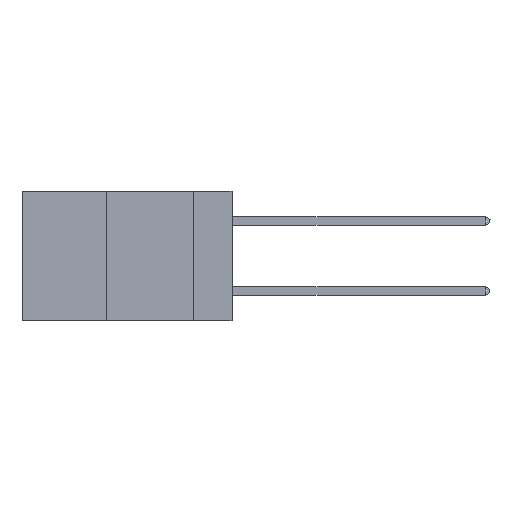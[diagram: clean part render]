
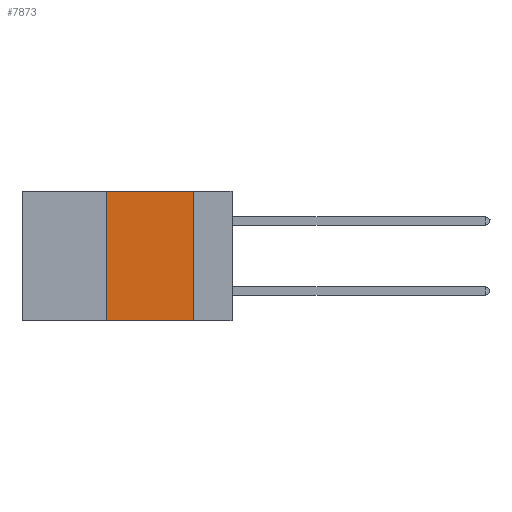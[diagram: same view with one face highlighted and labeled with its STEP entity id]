
A CAD part, left-side view. The second image highlights one B-rep face of the part: STEP entity #7873.
In plain terms, the highlighted planar face has unit normal (-1, 0, 0).
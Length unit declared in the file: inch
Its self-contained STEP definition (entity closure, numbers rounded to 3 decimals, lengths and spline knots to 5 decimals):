
#1733 = FACE_OUTER_BOUND ( 'NONE', #18670, .T. ) ;
#2161 = EDGE_CURVE ( 'NONE', #10029, #17665, #4350, .T. ) ;
#2415 = CARTESIAN_POINT ( 'NONE',  ( 0., 0.36, 0. ) ) ;
#2503 = VECTOR ( 'NONE', #9986, 39.37008 ) ;
#3212 = EDGE_CURVE ( 'NONE', #19777, #14713, #19995, .T. ) ;
#4350 = LINE ( 'NONE', #12884, #15622 ) ;
#5806 = LINE ( 'NONE', #18628, #14796 ) ;
#6129 = CARTESIAN_POINT ( 'NONE',  ( 0., 0.11, 0. ) ) ;
#6777 = CARTESIAN_POINT ( 'NONE',  ( 0., 0.11, 0. ) ) ;
#7456 = DIRECTION ( 'NONE',  ( 0., -1., 0. ) ) ;
#7873 = ADVANCED_FACE ( 'NONE', ( #1733 ), #9247, .F. ) ;
#9103 = ORIENTED_EDGE ( 'NONE', *, *, #13889, .T. ) ;
#9142 = CARTESIAN_POINT ( 'NONE',  ( 0., 0.6, -0.37 ) ) ;
#9247 = PLANE ( 'NONE',  #9894 ) ;
#9363 = EDGE_CURVE ( 'NONE', #17665, #19777, #5806, .T. ) ;
#9862 = ORIENTED_EDGE ( 'NONE', *, *, #3212, .F. ) ;
#9894 = AXIS2_PLACEMENT_3D ( 'NONE', #20603, #20751, #19154 ) ;
#9986 = DIRECTION ( 'NONE',  ( 0., 0., -1. ) ) ;
#9998 = LINE ( 'NONE', #9142, #17915 ) ;
#10029 = VERTEX_POINT ( 'NONE', #16297 ) ;
#12884 = CARTESIAN_POINT ( 'NONE',  ( 0., 0.36, 0. ) ) ;
#13889 = EDGE_CURVE ( 'NONE', #10029, #14713, #9998, .T. ) ;
#14054 = DIRECTION ( 'NONE',  ( 0., -1., 0. ) ) ;
#14384 = CARTESIAN_POINT ( 'NONE',  ( 0., 0.11, -0.37 ) ) ;
#14395 = DIRECTION ( 'NONE',  ( 0., 0., 1. ) ) ;
#14713 = VERTEX_POINT ( 'NONE', #14384 ) ;
#14796 = VECTOR ( 'NONE', #7456, 39.37008 ) ;
#14907 = ORIENTED_EDGE ( 'NONE', *, *, #9363, .F. ) ;
#15622 = VECTOR ( 'NONE', #14395, 39.37008 ) ;
#16297 = CARTESIAN_POINT ( 'NONE',  ( 0., 0.36, -0.37 ) ) ;
#17665 = VERTEX_POINT ( 'NONE', #2415 ) ;
#17915 = VECTOR ( 'NONE', #14054, 39.37008 ) ;
#18367 = ORIENTED_EDGE ( 'NONE', *, *, #2161, .F. ) ;
#18628 = CARTESIAN_POINT ( 'NONE',  ( 0., 0.6, 0. ) ) ;
#18670 = EDGE_LOOP ( 'NONE', ( #9862, #14907, #18367, #9103 ) ) ;
#19154 = DIRECTION ( 'NONE',  ( 0., 0., -1. ) ) ;
#19777 = VERTEX_POINT ( 'NONE', #6777 ) ;
#19995 = LINE ( 'NONE', #6129, #2503 ) ;
#20603 = CARTESIAN_POINT ( 'NONE',  ( 0., 0.6, 0. ) ) ;
#20751 = DIRECTION ( 'NONE',  ( 1., 0., 0. ) ) ;
